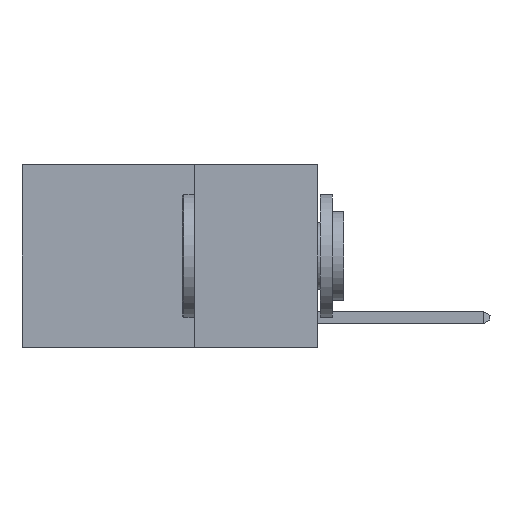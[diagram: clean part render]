
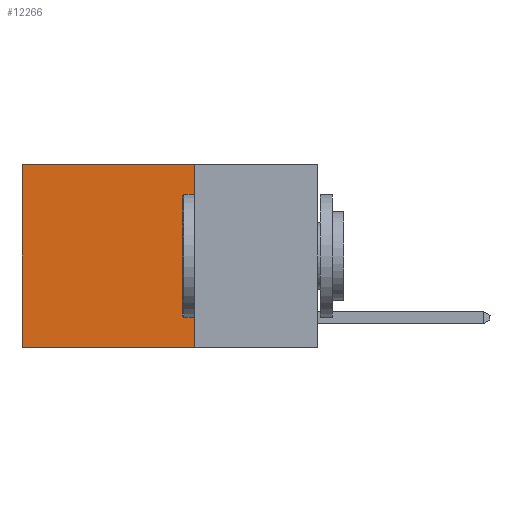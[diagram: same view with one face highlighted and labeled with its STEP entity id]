
A CAD part, left-side view. The second image highlights one B-rep face of the part: STEP entity #12266.
In plain terms, the highlighted planar face has unit normal (-1, 0, 0).
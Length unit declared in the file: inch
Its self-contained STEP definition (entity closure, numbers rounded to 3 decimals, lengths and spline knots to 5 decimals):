
#287 = CARTESIAN_POINT ( 'NONE',  ( 0.2625, 0.25, 0. ) ) ;
#940 = VECTOR ( 'NONE', #25864, 39.37008 ) ;
#1248 = ORIENTED_EDGE ( 'NONE', *, *, #17838, .T. ) ;
#1606 = LINE ( 'NONE', #13867, #940 ) ;
#1998 = CARTESIAN_POINT ( 'NONE',  ( 0.2625, 0.25, 0. ) ) ;
#2013 = VERTEX_POINT ( 'NONE', #1998 ) ;
#2336 = VECTOR ( 'NONE', #8425, 39.37008 ) ;
#3314 = DIRECTION ( 'NONE',  ( 0., 0., -1. ) ) ;
#3866 = VECTOR ( 'NONE', #12566, 39.37008 ) ;
#4556 = VERTEX_POINT ( 'NONE', #5152 ) ;
#4936 = VERTEX_POINT ( 'NONE', #16511 ) ;
#5152 = CARTESIAN_POINT ( 'NONE',  ( 0.2625, 0.25, -0.37 ) ) ;
#5180 = FACE_OUTER_BOUND ( 'NONE', #24661, .T. ) ;
#6602 = EDGE_CURVE ( 'NONE', #4556, #4936, #1606, .T. ) ;
#7370 = DIRECTION ( 'NONE',  ( 1., 0., 0. ) ) ;
#8129 = ORIENTED_EDGE ( 'NONE', *, *, #13153, .T. ) ;
#8425 = DIRECTION ( 'NONE',  ( 0., 0., -1. ) ) ;
#12266 = ADVANCED_FACE ( 'NONE', ( #5180 ), #15451, .F. ) ;
#12566 = DIRECTION ( 'NONE',  ( 0., 1., 0. ) ) ;
#12915 = EDGE_CURVE ( 'NONE', #2013, #4556, #25656, .T. ) ;
#13153 = EDGE_CURVE ( 'NONE', #2013, #13874, #14665, .T. ) ;
#13867 = CARTESIAN_POINT ( 'NONE',  ( 0.2625, 0.25, -0.37 ) ) ;
#13874 = VERTEX_POINT ( 'NONE', #23007 ) ;
#14665 = LINE ( 'NONE', #287, #3866 ) ;
#15451 = PLANE ( 'NONE',  #16915 ) ;
#15491 = CARTESIAN_POINT ( 'NONE',  ( 0.2625, 0.25, 0. ) ) ;
#16033 = ORIENTED_EDGE ( 'NONE', *, *, #6602, .F. ) ;
#16511 = CARTESIAN_POINT ( 'NONE',  ( 0.2625, 0.6, -0.37 ) ) ;
#16915 = AXIS2_PLACEMENT_3D ( 'NONE', #19542, #7370, #21538 ) ;
#17838 = EDGE_CURVE ( 'NONE', #13874, #4936, #17946, .T. ) ;
#17946 = LINE ( 'NONE', #20553, #2336 ) ;
#19224 = ORIENTED_EDGE ( 'NONE', *, *, #12915, .F. ) ;
#19542 = CARTESIAN_POINT ( 'NONE',  ( 0.2625, 0.25, 0. ) ) ;
#20553 = CARTESIAN_POINT ( 'NONE',  ( 0.2625, 0.6, 0. ) ) ;
#21538 = DIRECTION ( 'NONE',  ( 0., 0., -1. ) ) ;
#21622 = VECTOR ( 'NONE', #3314, 39.37008 ) ;
#23007 = CARTESIAN_POINT ( 'NONE',  ( 0.2625, 0.6, 0. ) ) ;
#24661 = EDGE_LOOP ( 'NONE', ( #1248, #16033, #19224, #8129 ) ) ;
#25656 = LINE ( 'NONE', #15491, #21622 ) ;
#25864 = DIRECTION ( 'NONE',  ( 0., 1., 0. ) ) ;
